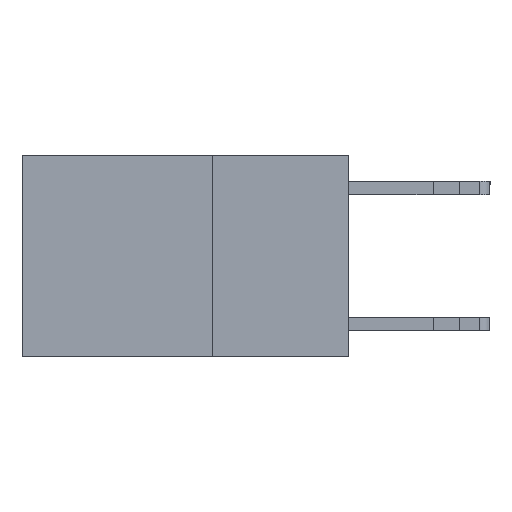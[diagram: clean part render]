
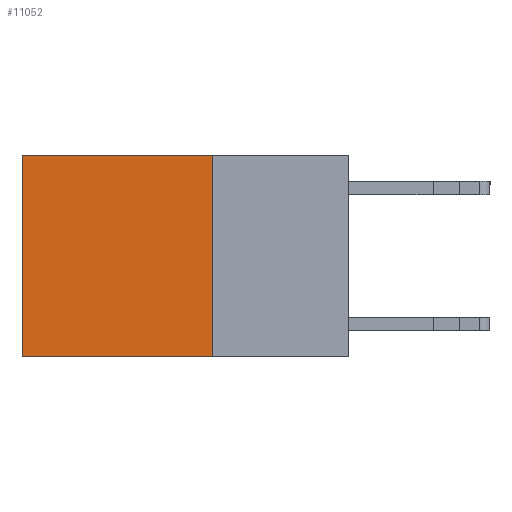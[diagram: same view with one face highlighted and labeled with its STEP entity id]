
A CAD part, left-side view. The second image highlights one B-rep face of the part: STEP entity #11052.
In plain terms, the highlighted planar face has unit normal (-1, 0, 0).
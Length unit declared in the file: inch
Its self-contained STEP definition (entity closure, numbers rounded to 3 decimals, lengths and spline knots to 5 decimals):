
#221 = LINE ( 'NONE', #8108, #10296 ) ;
#1192 = EDGE_CURVE ( 'NONE', #2779, #4471, #221, .T. ) ;
#1836 = LINE ( 'NONE', #16756, #17387 ) ;
#2706 = ORIENTED_EDGE ( 'NONE', *, *, #7108, .T. ) ;
#2715 = CARTESIAN_POINT ( 'NONE',  ( 0.2625, 0.25, 0. ) ) ;
#2779 = VERTEX_POINT ( 'NONE', #15881 ) ;
#2784 = EDGE_CURVE ( 'NONE', #4471, #10260, #4038, .T. ) ;
#2800 = LINE ( 'NONE', #8222, #8673 ) ;
#3685 = CARTESIAN_POINT ( 'NONE',  ( 0.2625, 0.25, -0.37 ) ) ;
#4038 = LINE ( 'NONE', #3685, #16515 ) ;
#4471 = VERTEX_POINT ( 'NONE', #7141 ) ;
#4565 = DIRECTION ( 'NONE',  ( 0., 0., -1. ) ) ;
#4956 = CARTESIAN_POINT ( 'NONE',  ( 0.2625, 0.6, -0.37 ) ) ;
#4989 = VERTEX_POINT ( 'NONE', #12524 ) ;
#5380 = DIRECTION ( 'NONE',  ( 0., 0., -1. ) ) ;
#6361 = DIRECTION ( 'NONE',  ( 0., 1., 0. ) ) ;
#6878 = ORIENTED_EDGE ( 'NONE', *, *, #11075, .T. ) ;
#7108 = EDGE_CURVE ( 'NONE', #4989, #10260, #1836, .T. ) ;
#7141 = CARTESIAN_POINT ( 'NONE',  ( 0.2625, 0.25, -0.37 ) ) ;
#8035 = DIRECTION ( 'NONE',  ( 1., 0., 0. ) ) ;
#8108 = CARTESIAN_POINT ( 'NONE',  ( 0.2625, 0.25, 0. ) ) ;
#8222 = CARTESIAN_POINT ( 'NONE',  ( 0.2625, 0.25, 0. ) ) ;
#8508 = ORIENTED_EDGE ( 'NONE', *, *, #2784, .F. ) ;
#8673 = VECTOR ( 'NONE', #15167, 39.37008 ) ;
#10260 = VERTEX_POINT ( 'NONE', #4956 ) ;
#10296 = VECTOR ( 'NONE', #13555, 39.37008 ) ;
#10996 = FACE_OUTER_BOUND ( 'NONE', #13607, .T. ) ;
#11052 = ADVANCED_FACE ( 'NONE', ( #10996 ), #14988, .F. ) ;
#11075 = EDGE_CURVE ( 'NONE', #2779, #4989, #2800, .T. ) ;
#12376 = AXIS2_PLACEMENT_3D ( 'NONE', #2715, #8035, #5380 ) ;
#12524 = CARTESIAN_POINT ( 'NONE',  ( 0.2625, 0.6, 0. ) ) ;
#13555 = DIRECTION ( 'NONE',  ( 0., 0., -1. ) ) ;
#13607 = EDGE_LOOP ( 'NONE', ( #2706, #8508, #15138, #6878 ) ) ;
#14988 = PLANE ( 'NONE',  #12376 ) ;
#15138 = ORIENTED_EDGE ( 'NONE', *, *, #1192, .F. ) ;
#15167 = DIRECTION ( 'NONE',  ( 0., 1., 0. ) ) ;
#15881 = CARTESIAN_POINT ( 'NONE',  ( 0.2625, 0.25, 0. ) ) ;
#16515 = VECTOR ( 'NONE', #6361, 39.37008 ) ;
#16756 = CARTESIAN_POINT ( 'NONE',  ( 0.2625, 0.6, 0. ) ) ;
#17387 = VECTOR ( 'NONE', #4565, 39.37008 ) ;
